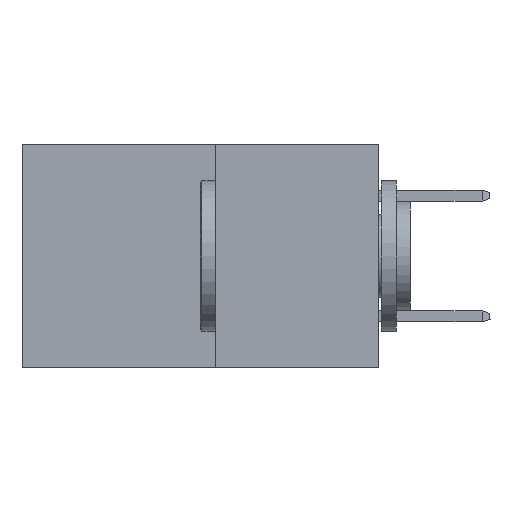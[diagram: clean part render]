
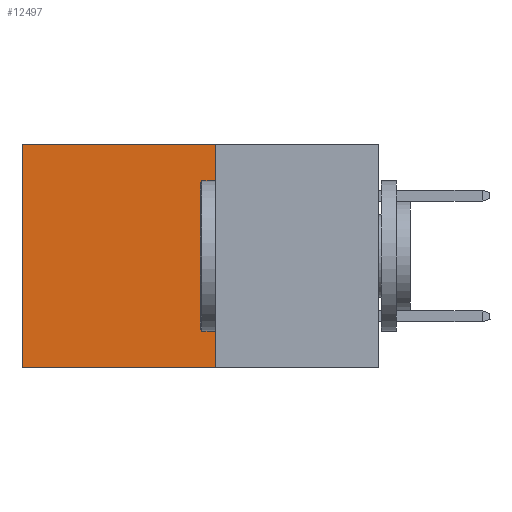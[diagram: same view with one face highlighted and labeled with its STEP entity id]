
A CAD part, left-side view. The second image highlights one B-rep face of the part: STEP entity #12497.
In plain terms, the highlighted planar face has unit normal (-1, 0, 0).
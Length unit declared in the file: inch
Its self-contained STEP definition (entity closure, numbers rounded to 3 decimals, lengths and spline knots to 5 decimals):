
#1157 = DIRECTION ( 'NONE',  ( 0., 1., 0. ) ) ;
#1830 = VERTEX_POINT ( 'NONE', #11175 ) ;
#1950 = ORIENTED_EDGE ( 'NONE', *, *, #8684, .T. ) ;
#3124 = LINE ( 'NONE', #21053, #20168 ) ;
#3288 = LINE ( 'NONE', #18274, #13980 ) ;
#3650 = EDGE_CURVE ( 'NONE', #5879, #17529, #4037, .T. ) ;
#4037 = LINE ( 'NONE', #20335, #21062 ) ;
#4216 = CARTESIAN_POINT ( 'NONE',  ( 0.277, 0.27, 0. ) ) ;
#5000 = ORIENTED_EDGE ( 'NONE', *, *, #20418, .F. ) ;
#5879 = VERTEX_POINT ( 'NONE', #4216 ) ;
#5960 = CARTESIAN_POINT ( 'NONE',  ( 0.277, 0.59, 0. ) ) ;
#7113 = CARTESIAN_POINT ( 'NONE',  ( 0.277, 0.27, 0. ) ) ;
#7643 = PLANE ( 'NONE',  #11110 ) ;
#7946 = FACE_OUTER_BOUND ( 'NONE', #12116, .T. ) ;
#8441 = VECTOR ( 'NONE', #15727, 39.37008 ) ;
#8684 = EDGE_CURVE ( 'NONE', #5879, #18767, #25491, .T. ) ;
#9703 = CARTESIAN_POINT ( 'NONE',  ( 0.277, 0.27, -0.37 ) ) ;
#9796 = DIRECTION ( 'NONE',  ( 0., 0., -1. ) ) ;
#10732 = ORIENTED_EDGE ( 'NONE', *, *, #17505, .T. ) ;
#11110 = AXIS2_PLACEMENT_3D ( 'NONE', #9703, #22585, #9796 ) ;
#11175 = CARTESIAN_POINT ( 'NONE',  ( 0.277, 0.59, -0.37 ) ) ;
#12116 = EDGE_LOOP ( 'NONE', ( #10732, #5000, #23870, #1950 ) ) ;
#12497 = ADVANCED_FACE ( 'NONE', ( #7946 ), #7643, .F. ) ;
#13980 = VECTOR ( 'NONE', #1157, 39.37008 ) ;
#15727 = DIRECTION ( 'NONE',  ( 0., 1., 0. ) ) ;
#17036 = CARTESIAN_POINT ( 'NONE',  ( 0.277, 0.27, -0.37 ) ) ;
#17505 = EDGE_CURVE ( 'NONE', #18767, #1830, #3124, .T. ) ;
#17529 = VERTEX_POINT ( 'NONE', #17036 ) ;
#18274 = CARTESIAN_POINT ( 'NONE',  ( 0.277, 0.27, -0.37 ) ) ;
#18767 = VERTEX_POINT ( 'NONE', #5960 ) ;
#19962 = DIRECTION ( 'NONE',  ( 0., 0., -1. ) ) ;
#20168 = VECTOR ( 'NONE', #21238, 39.37008 ) ;
#20335 = CARTESIAN_POINT ( 'NONE',  ( 0.277, 0.27, -0.37 ) ) ;
#20418 = EDGE_CURVE ( 'NONE', #17529, #1830, #3288, .T. ) ;
#21053 = CARTESIAN_POINT ( 'NONE',  ( 0.277, 0.59, -0.37 ) ) ;
#21062 = VECTOR ( 'NONE', #19962, 39.37008 ) ;
#21238 = DIRECTION ( 'NONE',  ( 0., 0., -1. ) ) ;
#22585 = DIRECTION ( 'NONE',  ( 1., 0., 0. ) ) ;
#23870 = ORIENTED_EDGE ( 'NONE', *, *, #3650, .F. ) ;
#25491 = LINE ( 'NONE', #7113, #8441 ) ;
